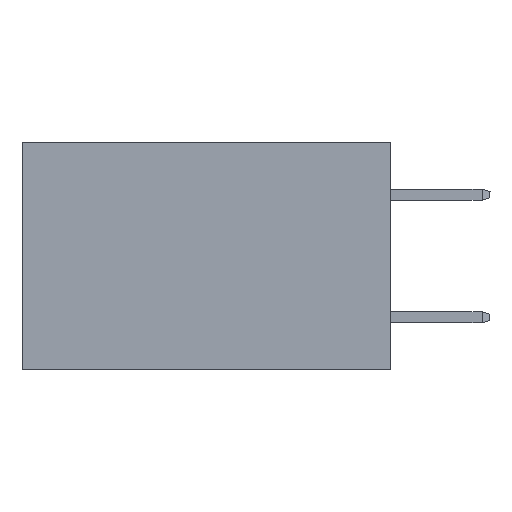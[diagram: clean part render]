
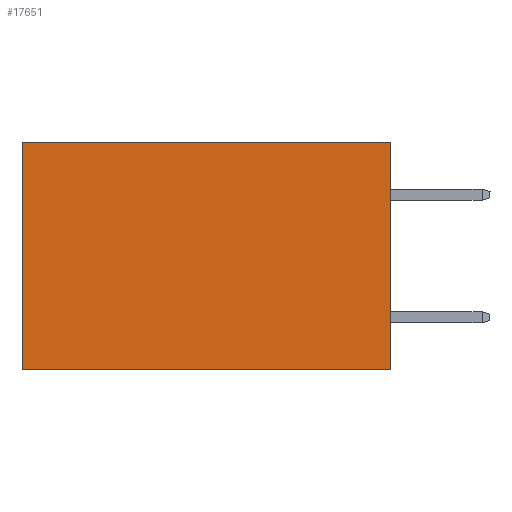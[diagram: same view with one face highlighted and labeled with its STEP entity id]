
A CAD part, left-side view. The second image highlights one B-rep face of the part: STEP entity #17651.
In plain terms, the highlighted planar face has unit normal (-1, 0, 0).
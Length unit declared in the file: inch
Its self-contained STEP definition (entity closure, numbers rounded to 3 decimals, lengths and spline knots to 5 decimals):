
#325 = EDGE_CURVE ( 'NONE', #9550, #2955, #13419, .T. ) ;
#940 = CARTESIAN_POINT ( 'NONE',  ( 0.2875, 0., -0.37 ) ) ;
#1821 = VERTEX_POINT ( 'NONE', #7760 ) ;
#2119 = VECTOR ( 'NONE', #4091, 39.37008 ) ;
#2955 = VERTEX_POINT ( 'NONE', #15713 ) ;
#3788 = PLANE ( 'NONE',  #8474 ) ;
#4091 = DIRECTION ( 'NONE',  ( 0., 0., -1. ) ) ;
#5094 = DIRECTION ( 'NONE',  ( 0., 0., -1. ) ) ;
#5236 = DIRECTION ( 'NONE',  ( 1., 0., 0. ) ) ;
#5492 = VECTOR ( 'NONE', #17497, 39.37008 ) ;
#6017 = DIRECTION ( 'NONE',  ( 0., 1., 0. ) ) ;
#6226 = VERTEX_POINT ( 'NONE', #8678 ) ;
#6299 = VECTOR ( 'NONE', #6017, 39.37008 ) ;
#6330 = CARTESIAN_POINT ( 'NONE',  ( 0.2875, 0.6, 0. ) ) ;
#6442 = LINE ( 'NONE', #10865, #2119 ) ;
#7760 = CARTESIAN_POINT ( 'NONE',  ( 0.2875, 0.6, 0. ) ) ;
#8043 = EDGE_LOOP ( 'NONE', ( #17032, #8350, #10200, #11198 ) ) ;
#8350 = ORIENTED_EDGE ( 'NONE', *, *, #325, .F. ) ;
#8474 = AXIS2_PLACEMENT_3D ( 'NONE', #9468, #5236, #14659 ) ;
#8678 = CARTESIAN_POINT ( 'NONE',  ( 0.2875, 0., 0. ) ) ;
#9468 = CARTESIAN_POINT ( 'NONE',  ( 0.2875, 0., 0. ) ) ;
#9550 = VERTEX_POINT ( 'NONE', #940 ) ;
#10200 = ORIENTED_EDGE ( 'NONE', *, *, #17779, .F. ) ;
#10226 = EDGE_CURVE ( 'NONE', #6226, #1821, #10467, .T. ) ;
#10467 = LINE ( 'NONE', #11995, #5492 ) ;
#10865 = CARTESIAN_POINT ( 'NONE',  ( 0.2875, 0., 0. ) ) ;
#11198 = ORIENTED_EDGE ( 'NONE', *, *, #10226, .T. ) ;
#11710 = CARTESIAN_POINT ( 'NONE',  ( 0.2875, 0., -0.37 ) ) ;
#11995 = CARTESIAN_POINT ( 'NONE',  ( 0.2875, 0., 0. ) ) ;
#13419 = LINE ( 'NONE', #11710, #6299 ) ;
#13794 = FACE_OUTER_BOUND ( 'NONE', #8043, .T. ) ;
#14157 = VECTOR ( 'NONE', #5094, 39.37008 ) ;
#14382 = LINE ( 'NONE', #6330, #14157 ) ;
#14659 = DIRECTION ( 'NONE',  ( 0., 0., -1. ) ) ;
#14677 = EDGE_CURVE ( 'NONE', #1821, #2955, #14382, .T. ) ;
#15713 = CARTESIAN_POINT ( 'NONE',  ( 0.2875, 0.6, -0.37 ) ) ;
#17032 = ORIENTED_EDGE ( 'NONE', *, *, #14677, .T. ) ;
#17497 = DIRECTION ( 'NONE',  ( 0., 1., 0. ) ) ;
#17651 = ADVANCED_FACE ( 'NONE', ( #13794 ), #3788, .F. ) ;
#17779 = EDGE_CURVE ( 'NONE', #6226, #9550, #6442, .T. ) ;
